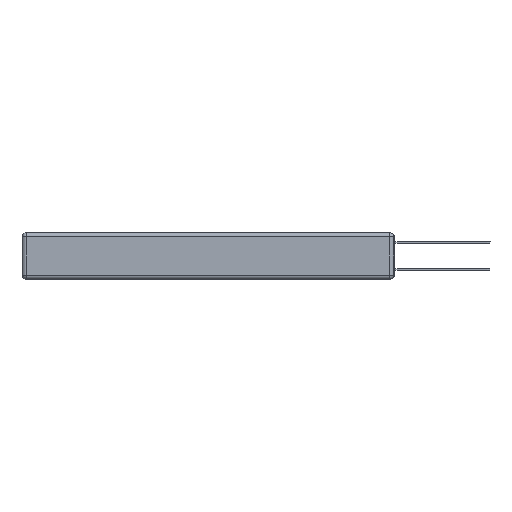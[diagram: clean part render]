
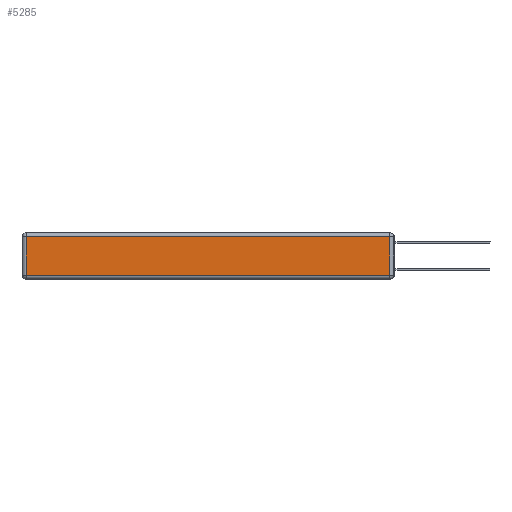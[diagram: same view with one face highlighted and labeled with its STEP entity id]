
A CAD part, left-side view. The second image highlights one B-rep face of the part: STEP entity #5285.
In plain terms, the highlighted planar face has unit normal (-1, 0, 0).
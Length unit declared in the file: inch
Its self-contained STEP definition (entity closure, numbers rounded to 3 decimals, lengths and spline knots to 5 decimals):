
#357 = DIRECTION ( 'NONE',  ( 0., 0., 1. ) ) ;
#469 = EDGE_CURVE ( 'NONE', #7317, #5972, #7472, .T. ) ;
#1024 = VECTOR ( 'NONE', #6246, 39.37008 ) ;
#1220 = DIRECTION ( 'NONE',  ( 0., 0., 1. ) ) ;
#1398 = VECTOR ( 'NONE', #8711, 39.37008 ) ;
#1494 = CARTESIAN_POINT ( 'NONE',  ( 0., 0.03, -0.03 ) ) ;
#1694 = EDGE_CURVE ( 'NONE', #9891, #7317, #9422, .T. ) ;
#1716 = ORIENTED_EDGE ( 'NONE', *, *, #469, .T. ) ;
#1778 = AXIS2_PLACEMENT_3D ( 'NONE', #12857, #12722, #357 ) ;
#2301 = CARTESIAN_POINT ( 'NONE',  ( 0., 0.03, -0.313 ) ) ;
#3434 = CARTESIAN_POINT ( 'NONE',  ( 0., 2.72, -0.313 ) ) ;
#3495 = VERTEX_POINT ( 'NONE', #3434 ) ;
#3595 = FACE_OUTER_BOUND ( 'NONE', #3919, .T. ) ;
#3919 = EDGE_LOOP ( 'NONE', ( #4685, #5844, #1716, #6987 ) ) ;
#4685 = ORIENTED_EDGE ( 'NONE', *, *, #12525, .T. ) ;
#5285 = ADVANCED_FACE ( 'NONE', ( #3595 ), #8828, .T. ) ;
#5769 = LINE ( 'NONE', #12871, #1398 ) ;
#5844 = ORIENTED_EDGE ( 'NONE', *, *, #1694, .T. ) ;
#5972 = VERTEX_POINT ( 'NONE', #6871 ) ;
#6223 = VECTOR ( 'NONE', #1220, 39.37008 ) ;
#6246 = DIRECTION ( 'NONE',  ( 0., -1., 0. ) ) ;
#6442 = CARTESIAN_POINT ( 'NONE',  ( 0., 0., -0.313 ) ) ;
#6871 = CARTESIAN_POINT ( 'NONE',  ( 0., 2.72, -0.03 ) ) ;
#6987 = ORIENTED_EDGE ( 'NONE', *, *, #10696, .T. ) ;
#7317 = VERTEX_POINT ( 'NONE', #1494 ) ;
#7472 = LINE ( 'NONE', #11697, #11640 ) ;
#8711 = DIRECTION ( 'NONE',  ( 0., 0., -1. ) ) ;
#8828 = PLANE ( 'NONE',  #1778 ) ;
#9167 = CARTESIAN_POINT ( 'NONE',  ( 0., 0.03, -0.343 ) ) ;
#9422 = LINE ( 'NONE', #9167, #6223 ) ;
#9891 = VERTEX_POINT ( 'NONE', #2301 ) ;
#10325 = LINE ( 'NONE', #6442, #1024 ) ;
#10696 = EDGE_CURVE ( 'NONE', #5972, #3495, #5769, .T. ) ;
#11640 = VECTOR ( 'NONE', #12576, 39.37008 ) ;
#11697 = CARTESIAN_POINT ( 'NONE',  ( 0., 2.75, -0.03 ) ) ;
#12525 = EDGE_CURVE ( 'NONE', #3495, #9891, #10325, .T. ) ;
#12576 = DIRECTION ( 'NONE',  ( 0., 1., 0. ) ) ;
#12722 = DIRECTION ( 'NONE',  ( -1., 0., 0. ) ) ;
#12857 = CARTESIAN_POINT ( 'NONE',  ( 0., 0., -0.343 ) ) ;
#12871 = CARTESIAN_POINT ( 'NONE',  ( 0., 2.72, -0.343 ) ) ;
